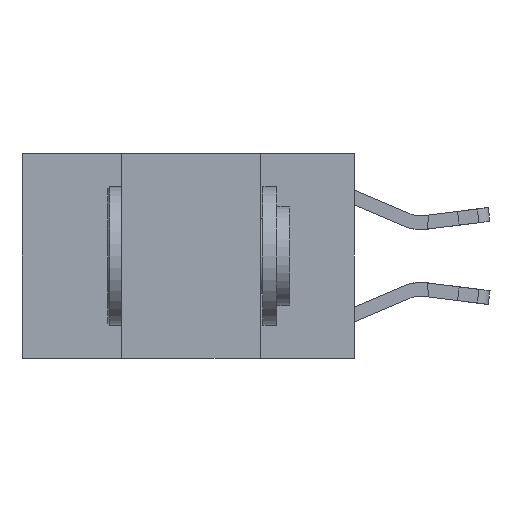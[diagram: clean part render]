
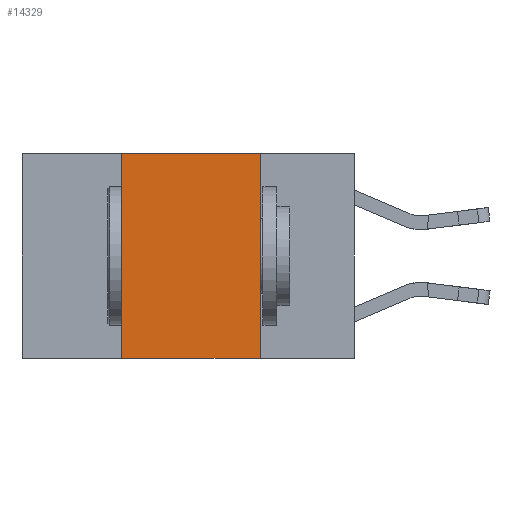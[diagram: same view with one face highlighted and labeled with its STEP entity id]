
A CAD part, left-side view. The second image highlights one B-rep face of the part: STEP entity #14329.
In plain terms, the highlighted planar face has unit normal (-1, 0, 0).
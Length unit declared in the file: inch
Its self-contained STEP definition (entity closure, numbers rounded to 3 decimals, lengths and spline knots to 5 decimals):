
#416 = VECTOR ( 'NONE', #13675, 39.37008 ) ;
#927 = ORIENTED_EDGE ( 'NONE', *, *, #6712, .F. ) ;
#1467 = CARTESIAN_POINT ( 'NONE',  ( 0., 0.17, -0.37 ) ) ;
#3084 = DIRECTION ( 'NONE',  ( 0., -1., 0. ) ) ;
#3173 = CARTESIAN_POINT ( 'NONE',  ( 0., 0.6, -0.37 ) ) ;
#3281 = ORIENTED_EDGE ( 'NONE', *, *, #15775, .F. ) ;
#3436 = VECTOR ( 'NONE', #3084, 39.37008 ) ;
#3798 = LINE ( 'NONE', #12147, #10660 ) ;
#3865 = LINE ( 'NONE', #9928, #3436 ) ;
#4127 = PLANE ( 'NONE',  #12855 ) ;
#5510 = DIRECTION ( 'NONE',  ( 0., 0., -1. ) ) ;
#6473 = CARTESIAN_POINT ( 'NONE',  ( 0., 0.17, 0. ) ) ;
#6712 = EDGE_CURVE ( 'NONE', #8492, #14349, #3798, .T. ) ;
#6948 = LINE ( 'NONE', #3173, #13254 ) ;
#6954 = EDGE_LOOP ( 'NONE', ( #3281, #10360, #927, #13862 ) ) ;
#8492 = VERTEX_POINT ( 'NONE', #11804 ) ;
#9081 = FACE_OUTER_BOUND ( 'NONE', #6954, .T. ) ;
#9588 = CARTESIAN_POINT ( 'NONE',  ( 0., 0.6, 0. ) ) ;
#9679 = EDGE_CURVE ( 'NONE', #8492, #12555, #6948, .T. ) ;
#9928 = CARTESIAN_POINT ( 'NONE',  ( 0., 0.6, 0. ) ) ;
#10012 = DIRECTION ( 'NONE',  ( 0., -1., 0. ) ) ;
#10307 = EDGE_CURVE ( 'NONE', #14349, #11290, #3865, .T. ) ;
#10360 = ORIENTED_EDGE ( 'NONE', *, *, #10307, .F. ) ;
#10660 = VECTOR ( 'NONE', #13485, 39.37008 ) ;
#11290 = VERTEX_POINT ( 'NONE', #6473 ) ;
#11368 = LINE ( 'NONE', #12328, #416 ) ;
#11804 = CARTESIAN_POINT ( 'NONE',  ( 0., 0.42, -0.37 ) ) ;
#12147 = CARTESIAN_POINT ( 'NONE',  ( 0., 0.42, 0. ) ) ;
#12328 = CARTESIAN_POINT ( 'NONE',  ( 0., 0.17, 0. ) ) ;
#12555 = VERTEX_POINT ( 'NONE', #1467 ) ;
#12855 = AXIS2_PLACEMENT_3D ( 'NONE', #9588, #13636, #5510 ) ;
#13254 = VECTOR ( 'NONE', #10012, 39.37008 ) ;
#13485 = DIRECTION ( 'NONE',  ( 0., 0., 1. ) ) ;
#13636 = DIRECTION ( 'NONE',  ( 1., 0., 0. ) ) ;
#13675 = DIRECTION ( 'NONE',  ( 0., 0., -1. ) ) ;
#13862 = ORIENTED_EDGE ( 'NONE', *, *, #9679, .T. ) ;
#14329 = ADVANCED_FACE ( 'NONE', ( #9081 ), #4127, .F. ) ;
#14349 = VERTEX_POINT ( 'NONE', #15046 ) ;
#15046 = CARTESIAN_POINT ( 'NONE',  ( 0., 0.42, 0. ) ) ;
#15775 = EDGE_CURVE ( 'NONE', #11290, #12555, #11368, .T. ) ;
